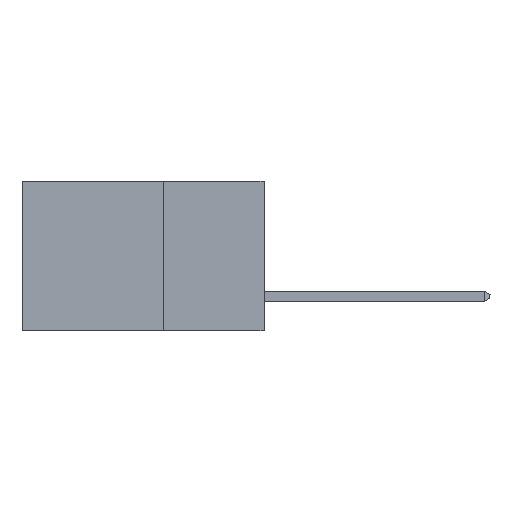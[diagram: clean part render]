
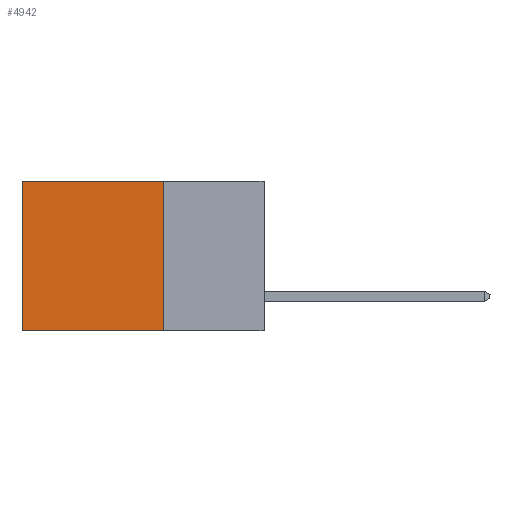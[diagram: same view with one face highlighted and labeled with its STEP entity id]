
A CAD part, left-side view. The second image highlights one B-rep face of the part: STEP entity #4942.
In plain terms, the highlighted planar face has unit normal (-1, 0, 0).
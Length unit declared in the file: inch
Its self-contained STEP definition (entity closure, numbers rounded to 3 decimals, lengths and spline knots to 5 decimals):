
#264 = VERTEX_POINT ( 'NONE', #851 ) ;
#473 = DIRECTION ( 'NONE',  ( 1., 0., 0. ) ) ;
#491 = EDGE_LOOP ( 'NONE', ( #6312, #7486, #6791, #3587 ) ) ;
#579 = DIRECTION ( 'NONE',  ( 0., 1., 0. ) ) ;
#851 = CARTESIAN_POINT ( 'NONE',  ( 0.2615, 0.25, 0. ) ) ;
#2031 = PLANE ( 'NONE',  #4585 ) ;
#2097 = EDGE_CURVE ( 'NONE', #4972, #4437, #7735, .T. ) ;
#2678 = CARTESIAN_POINT ( 'NONE',  ( 0.2615, 0.25, -0.37 ) ) ;
#3302 = VECTOR ( 'NONE', #8384, 39.37008 ) ;
#3443 = DIRECTION ( 'NONE',  ( 0., 0., -1. ) ) ;
#3587 = ORIENTED_EDGE ( 'NONE', *, *, #3984, .T. ) ;
#3984 = EDGE_CURVE ( 'NONE', #264, #9260, #9871, .T. ) ;
#4437 = VERTEX_POINT ( 'NONE', #8984 ) ;
#4491 = EDGE_CURVE ( 'NONE', #264, #4972, #7419, .T. ) ;
#4585 = AXIS2_PLACEMENT_3D ( 'NONE', #5214, #473, #5423 ) ;
#4942 = ADVANCED_FACE ( 'NONE', ( #6098 ), #2031, .F. ) ;
#4972 = VERTEX_POINT ( 'NONE', #9392 ) ;
#5094 = CARTESIAN_POINT ( 'NONE',  ( 0.2615, 0.6, -0.37 ) ) ;
#5214 = CARTESIAN_POINT ( 'NONE',  ( 0.2615, 0.25, -0.37 ) ) ;
#5423 = DIRECTION ( 'NONE',  ( 0., 0., -1. ) ) ;
#6098 = FACE_OUTER_BOUND ( 'NONE', #491, .T. ) ;
#6103 = CARTESIAN_POINT ( 'NONE',  ( 0.2615, 0.6, 0. ) ) ;
#6306 = CARTESIAN_POINT ( 'NONE',  ( 0.2615, 0.25, -0.37 ) ) ;
#6312 = ORIENTED_EDGE ( 'NONE', *, *, #7712, .T. ) ;
#6392 = VECTOR ( 'NONE', #579, 39.37008 ) ;
#6791 = ORIENTED_EDGE ( 'NONE', *, *, #4491, .F. ) ;
#7349 = LINE ( 'NONE', #5094, #8446 ) ;
#7419 = LINE ( 'NONE', #2678, #8066 ) ;
#7486 = ORIENTED_EDGE ( 'NONE', *, *, #2097, .F. ) ;
#7712 = EDGE_CURVE ( 'NONE', #9260, #4437, #7349, .T. ) ;
#7735 = LINE ( 'NONE', #6306, #6392 ) ;
#7749 = DIRECTION ( 'NONE',  ( 0., 0., -1. ) ) ;
#8066 = VECTOR ( 'NONE', #7749, 39.37008 ) ;
#8384 = DIRECTION ( 'NONE',  ( 0., 1., 0. ) ) ;
#8446 = VECTOR ( 'NONE', #3443, 39.37008 ) ;
#8984 = CARTESIAN_POINT ( 'NONE',  ( 0.2615, 0.6, -0.37 ) ) ;
#9165 = CARTESIAN_POINT ( 'NONE',  ( 0.2615, 0.25, 0. ) ) ;
#9260 = VERTEX_POINT ( 'NONE', #6103 ) ;
#9392 = CARTESIAN_POINT ( 'NONE',  ( 0.2615, 0.25, -0.37 ) ) ;
#9871 = LINE ( 'NONE', #9165, #3302 ) ;
